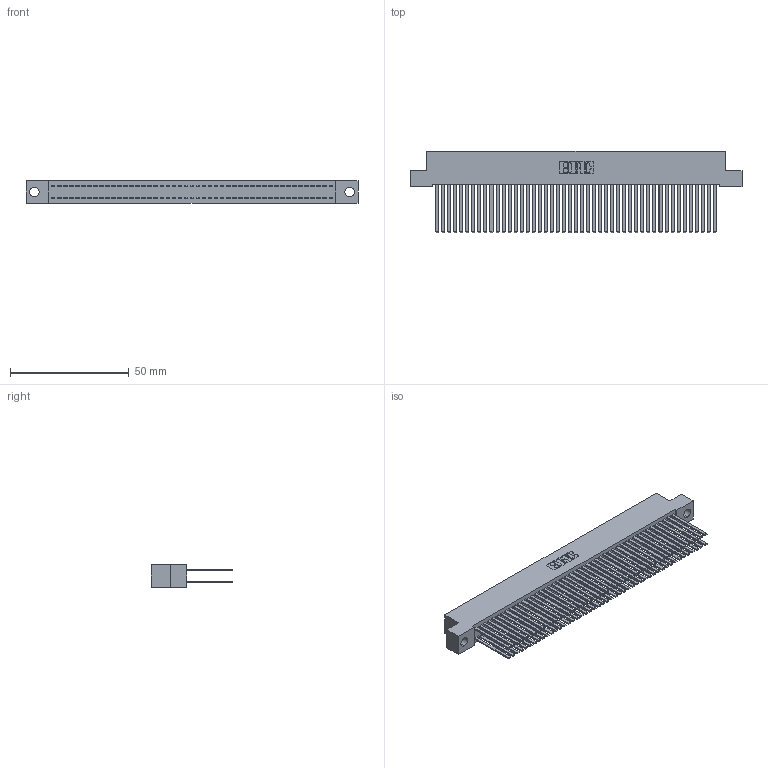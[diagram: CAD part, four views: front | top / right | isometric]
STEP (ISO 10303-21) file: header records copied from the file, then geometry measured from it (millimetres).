
FILE_DESCRIPTION (( 'STEP AP203' ), '1' );
FILE_NAME ('342-094-544-204.STEP', '2019-10-04T15:33:56', ( '' ), ( '' ), 'SwSTEP 2.0', 'SolidWorks 2016', '' );
FILE_SCHEMA (( 'CONFIG_CONTROL_DESIGN' ));
Length unit declared in the file: inch
Products named in the file (3): 342-094-544-204; 342 Part_.156 TH; 345-292-001_345-293-144
Assembly tree (95 placements, depth 2):
  342-094-544-204
    342 Part_.156 TH
    345-292-001_345-293-144  x94
Bounding box: 139.7 x 34.3 x 9.4 mm (x, y, z)
Volume: 13806.4 mm3; surface area: 26069.9 mm2
Topology: 95 solids, 95 shells, 4434 faces, 13177 edges, 8658 vertices
Faces by surface type: plane 3074, cylinder 1360
Entity records: 29277 total; most frequent: CARTESIAN_POINT 4842, ORIENTED_EDGE 4778, DIRECTION 4125, EDGE_CURVE 2389, LINE 2265, VECTOR 2265, VERTEX_POINT 1590, AXIS2_PLACEMENT_3D 930
